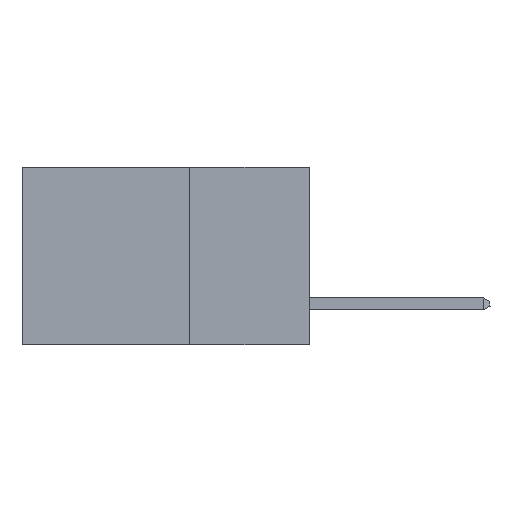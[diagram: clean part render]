
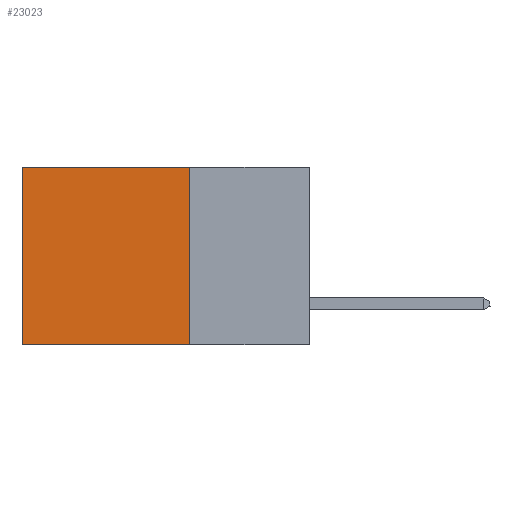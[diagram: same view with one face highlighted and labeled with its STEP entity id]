
A CAD part, left-side view. The second image highlights one B-rep face of the part: STEP entity #23023.
In plain terms, the highlighted planar face has unit normal (-1, 0, 0).
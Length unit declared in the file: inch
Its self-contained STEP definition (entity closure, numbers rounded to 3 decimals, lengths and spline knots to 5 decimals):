
#1190 = CARTESIAN_POINT ( 'NONE',  ( 0.2875, 0.25, 0. ) ) ;
#3132 = CARTESIAN_POINT ( 'NONE',  ( 0.2875, 0.25, 0. ) ) ;
#3215 = PLANE ( 'NONE',  #5807 ) ;
#3312 = LINE ( 'NONE', #1190, #17478 ) ;
#3375 = LINE ( 'NONE', #3132, #22245 ) ;
#3751 = CARTESIAN_POINT ( 'NONE',  ( 0.2875, 0.6, -0.37 ) ) ;
#4119 = CARTESIAN_POINT ( 'NONE',  ( 0.2875, 0.6, 0. ) ) ;
#4372 = CARTESIAN_POINT ( 'NONE',  ( 0.2875, 0.25, 0. ) ) ;
#5210 = EDGE_CURVE ( 'NONE', #7349, #13349, #5708, .T. ) ;
#5244 = DIRECTION ( 'NONE',  ( 0., 1., 0. ) ) ;
#5708 = LINE ( 'NONE', #7650, #11672 ) ;
#5724 = DIRECTION ( 'NONE',  ( 0., 0., -1. ) ) ;
#5807 = AXIS2_PLACEMENT_3D ( 'NONE', #15512, #7234, #17386 ) ;
#6708 = ORIENTED_EDGE ( 'NONE', *, *, #18447, .F. ) ;
#7234 = DIRECTION ( 'NONE',  ( 1., 0., 0. ) ) ;
#7349 = VERTEX_POINT ( 'NONE', #4119 ) ;
#7650 = CARTESIAN_POINT ( 'NONE',  ( 0.2875, 0.6, 0. ) ) ;
#8127 = DIRECTION ( 'NONE',  ( 0., 1., 0. ) ) ;
#8541 = CARTESIAN_POINT ( 'NONE',  ( 0.2875, 0.25, -0.37 ) ) ;
#9277 = ORIENTED_EDGE ( 'NONE', *, *, #5210, .T. ) ;
#10087 = EDGE_LOOP ( 'NONE', ( #9277, #13482, #6708, #14057 ) ) ;
#11672 = VECTOR ( 'NONE', #21553, 39.37008 ) ;
#12365 = VERTEX_POINT ( 'NONE', #8541 ) ;
#12405 = LINE ( 'NONE', #17993, #15559 ) ;
#12819 = VERTEX_POINT ( 'NONE', #4372 ) ;
#13349 = VERTEX_POINT ( 'NONE', #3751 ) ;
#13482 = ORIENTED_EDGE ( 'NONE', *, *, #25148, .F. ) ;
#14057 = ORIENTED_EDGE ( 'NONE', *, *, #23141, .T. ) ;
#15512 = CARTESIAN_POINT ( 'NONE',  ( 0.2875, 0.25, 0. ) ) ;
#15559 = VECTOR ( 'NONE', #8127, 39.37008 ) ;
#16928 = FACE_OUTER_BOUND ( 'NONE', #10087, .T. ) ;
#17386 = DIRECTION ( 'NONE',  ( 0., 0., -1. ) ) ;
#17478 = VECTOR ( 'NONE', #5724, 39.37008 ) ;
#17993 = CARTESIAN_POINT ( 'NONE',  ( 0.2875, 0.25, -0.37 ) ) ;
#18447 = EDGE_CURVE ( 'NONE', #12819, #12365, #3312, .T. ) ;
#21553 = DIRECTION ( 'NONE',  ( 0., 0., -1. ) ) ;
#22245 = VECTOR ( 'NONE', #5244, 39.37008 ) ;
#23023 = ADVANCED_FACE ( 'NONE', ( #16928 ), #3215, .F. ) ;
#23141 = EDGE_CURVE ( 'NONE', #12819, #7349, #3375, .T. ) ;
#25148 = EDGE_CURVE ( 'NONE', #12365, #13349, #12405, .T. ) ;
